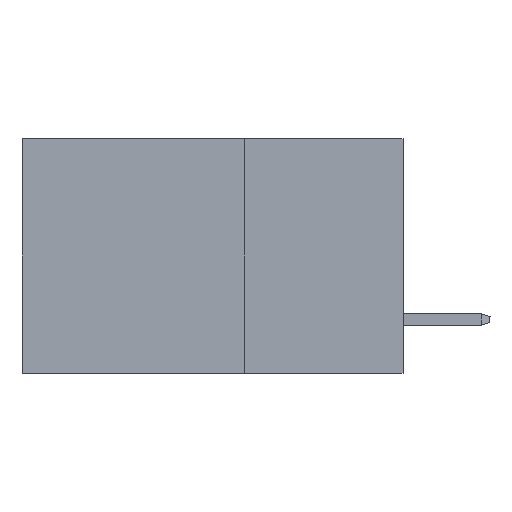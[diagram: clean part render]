
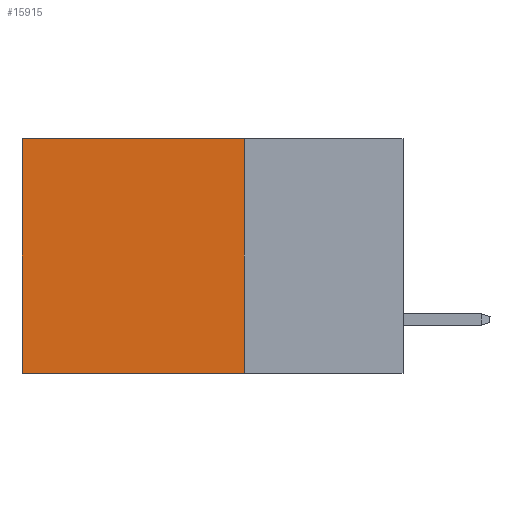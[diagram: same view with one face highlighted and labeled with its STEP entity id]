
A CAD part, left-side view. The second image highlights one B-rep face of the part: STEP entity #15915.
In plain terms, the highlighted planar face has unit normal (-1, 0, 0).
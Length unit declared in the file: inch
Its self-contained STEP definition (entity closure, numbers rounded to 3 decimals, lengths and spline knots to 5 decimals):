
#165 = VERTEX_POINT ( 'NONE', #24797 ) ;
#619 = LINE ( 'NONE', #13889, #23639 ) ;
#1200 = EDGE_CURVE ( 'NONE', #165, #9040, #17510, .T. ) ;
#1412 = VERTEX_POINT ( 'NONE', #16226 ) ;
#1591 = LINE ( 'NONE', #9176, #13654 ) ;
#2092 = ORIENTED_EDGE ( 'NONE', *, *, #11975, .F. ) ;
#3782 = ORIENTED_EDGE ( 'NONE', *, *, #1200, .T. ) ;
#5198 = CARTESIAN_POINT ( 'NONE',  ( 0.2875, 0.25, -0.37 ) ) ;
#5446 = ORIENTED_EDGE ( 'NONE', *, *, #31885, .T. ) ;
#6275 = DIRECTION ( 'NONE',  ( 0., 1., 0. ) ) ;
#6660 = CARTESIAN_POINT ( 'NONE',  ( 0.2875, 0.6, 0. ) ) ;
#8687 = CARTESIAN_POINT ( 'NONE',  ( 0.2875, 0.6, -0.37 ) ) ;
#9040 = VERTEX_POINT ( 'NONE', #8687 ) ;
#9176 = CARTESIAN_POINT ( 'NONE',  ( 0.2875, 0.25, -0.37 ) ) ;
#10408 = VERTEX_POINT ( 'NONE', #5198 ) ;
#11858 = FACE_OUTER_BOUND ( 'NONE', #20779, .T. ) ;
#11975 = EDGE_CURVE ( 'NONE', #10408, #9040, #1591, .T. ) ;
#12207 = LINE ( 'NONE', #17366, #22508 ) ;
#13654 = VECTOR ( 'NONE', #6275, 39.37008 ) ;
#13889 = CARTESIAN_POINT ( 'NONE',  ( 0.2875, 0.25, 0. ) ) ;
#15915 = ADVANCED_FACE ( 'NONE', ( #11858 ), #22346, .F. ) ;
#16226 = CARTESIAN_POINT ( 'NONE',  ( 0.2875, 0.25, 0. ) ) ;
#17154 = AXIS2_PLACEMENT_3D ( 'NONE', #32918, #19797, #20973 ) ;
#17366 = CARTESIAN_POINT ( 'NONE',  ( 0.2875, 0.25, 0. ) ) ;
#17510 = LINE ( 'NONE', #6660, #17834 ) ;
#17834 = VECTOR ( 'NONE', #19760, 39.37008 ) ;
#19760 = DIRECTION ( 'NONE',  ( 0., 0., -1. ) ) ;
#19797 = DIRECTION ( 'NONE',  ( 1., 0., 0. ) ) ;
#20779 = EDGE_LOOP ( 'NONE', ( #3782, #2092, #29007, #5446 ) ) ;
#20973 = DIRECTION ( 'NONE',  ( 0., 0., -1. ) ) ;
#22346 = PLANE ( 'NONE',  #17154 ) ;
#22508 = VECTOR ( 'NONE', #27912, 39.37008 ) ;
#23639 = VECTOR ( 'NONE', #27531, 39.37008 ) ;
#24797 = CARTESIAN_POINT ( 'NONE',  ( 0.2875, 0.6, 0. ) ) ;
#27531 = DIRECTION ( 'NONE',  ( 0., 1., 0. ) ) ;
#27912 = DIRECTION ( 'NONE',  ( 0., 0., -1. ) ) ;
#29007 = ORIENTED_EDGE ( 'NONE', *, *, #29777, .F. ) ;
#29777 = EDGE_CURVE ( 'NONE', #1412, #10408, #12207, .T. ) ;
#31885 = EDGE_CURVE ( 'NONE', #1412, #165, #619, .T. ) ;
#32918 = CARTESIAN_POINT ( 'NONE',  ( 0.2875, 0.25, 0. ) ) ;
